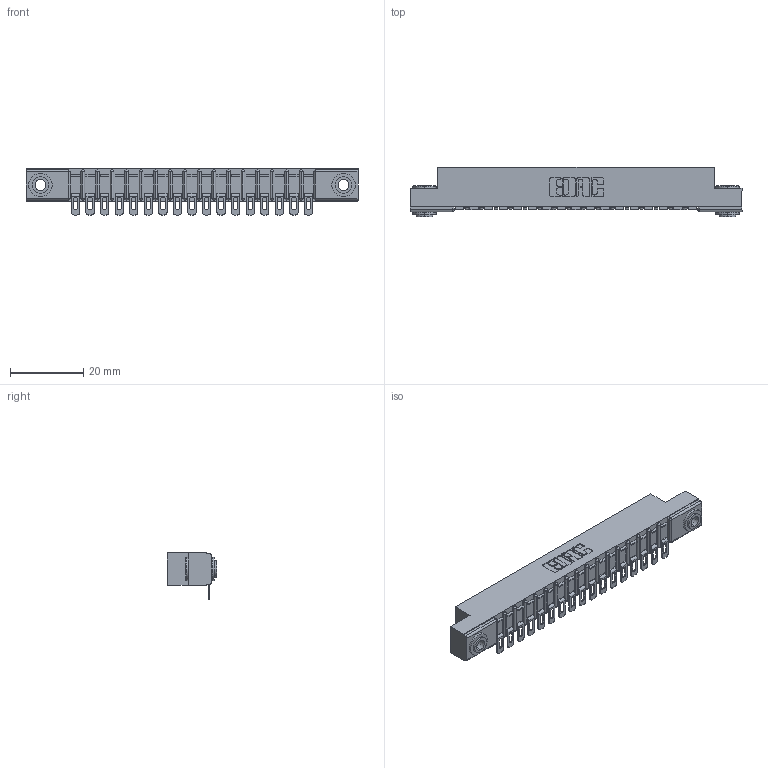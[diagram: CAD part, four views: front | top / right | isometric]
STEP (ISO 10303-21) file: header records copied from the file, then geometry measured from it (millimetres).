
FILE_DESCRIPTION (( 'STEP AP203' ), '1' );
FILE_NAME ('357-017-554-103.STEP', '2018-08-08T04:06:47', ( '' ), ( '' ), 'SwSTEP 2.0', 'SolidWorks 2016', '' );
FILE_SCHEMA (( 'CONFIG_CONTROL_DESIGN' ));
Length unit declared in the file: inch
Products named in the file (4): 345-250-002_345-250-002-102; 357-017-554-103; 307 Part_.156 Dia Mounting Holes; 307-290-002_554
Assembly tree (20 placements, depth 2):
  357-017-554-103
    307 Part_.156 Dia Mounting Holes
    307-290-002_554  x17
    345-250-002_345-250-002-102  x2
Bounding box: 90.37 x 13.36 x 12.52 mm (x, y, z)
Volume: 5971.1 mm3; surface area: 10896.2 mm2
Topology: 20 solids, 20 shells, 1565 faces, 4736 edges, 3104 vertices
Faces by surface type: plane 876, cylinder 645, sphere 36, cone 8
Entity records: 19686 total; most frequent: CARTESIAN_POINT 3295, ORIENTED_EDGE 3276, DIRECTION 3234, EDGE_CURVE 1638, LINE 1228, VECTOR 1228, VERTEX_POINT 1064, AXIS2_PLACEMENT_3D 1003
